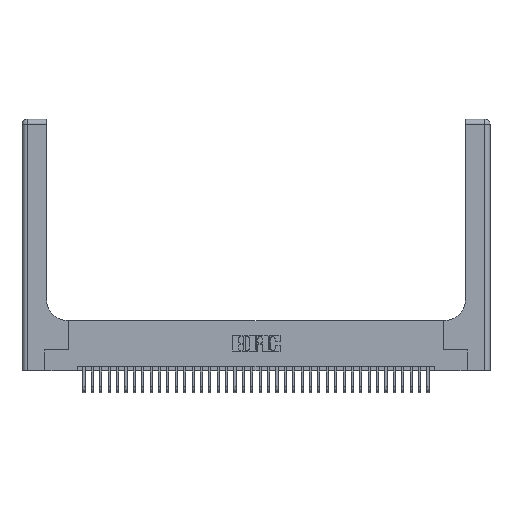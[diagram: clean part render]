
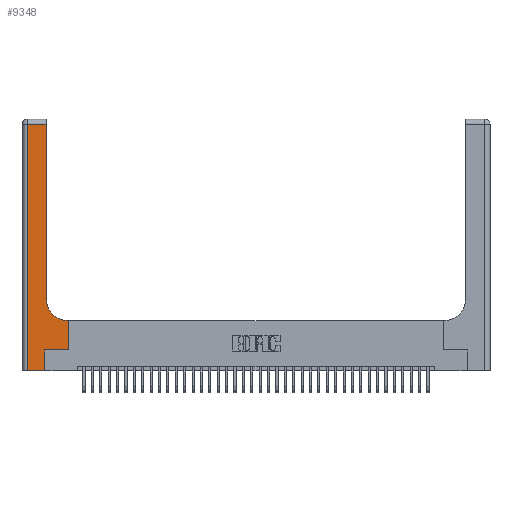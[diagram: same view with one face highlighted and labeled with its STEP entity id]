
A CAD part, top view. The second image highlights one B-rep face of the part: STEP entity #9348.
In plain terms, the highlighted planar face has unit normal (0, 0, 1).
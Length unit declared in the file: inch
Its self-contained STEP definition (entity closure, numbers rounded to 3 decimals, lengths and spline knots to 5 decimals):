
#837 = VECTOR ( 'NONE', #2666, 39.37008 ) ;
#990 = VECTOR ( 'NONE', #32367, 39.37008 ) ;
#1146 = CARTESIAN_POINT ( 'NONE',  ( 0.2915, 0.6, 0.37 ) ) ;
#1640 = CARTESIAN_POINT ( 'NONE',  ( 0., 3., 0.37 ) ) ;
#1773 = DIRECTION ( 'NONE',  ( 0., 0., -1. ) ) ;
#2666 = DIRECTION ( 'NONE',  ( 1., 0., 0. ) ) ;
#3474 = VERTEX_POINT ( 'NONE', #8706 ) ;
#3590 = CARTESIAN_POINT ( 'NONE',  ( 0.269, 0.25, 0.37 ) ) ;
#4107 = ORIENTED_EDGE ( 'NONE', *, *, #10324, .T. ) ;
#4126 = VERTEX_POINT ( 'NONE', #3590 ) ;
#4825 = DIRECTION ( 'NONE',  ( 0., 0., -1. ) ) ;
#5208 = ORIENTED_EDGE ( 'NONE', *, *, #34622, .T. ) ;
#5477 = DIRECTION ( 'NONE',  ( -1., 0., 0. ) ) ;
#5587 = EDGE_CURVE ( 'NONE', #35116, #32030, #19634, .T. ) ;
#6352 = ORIENTED_EDGE ( 'NONE', *, *, #35285, .T. ) ;
#6358 = VECTOR ( 'NONE', #16440, 39.37008 ) ;
#8196 = VECTOR ( 'NONE', #34169, 39.37008 ) ;
#8706 = CARTESIAN_POINT ( 'NONE',  ( 0.06, 2.94, 0.37 ) ) ;
#8717 = EDGE_CURVE ( 'NONE', #3474, #21425, #32733, .T. ) ;
#9348 = ADVANCED_FACE ( 'NONE', ( #12193 ), #35833, .F. ) ;
#9708 = VERTEX_POINT ( 'NONE', #20956 ) ;
#10324 = EDGE_CURVE ( 'NONE', #33354, #25528, #24553, .T. ) ;
#10590 = ORIENTED_EDGE ( 'NONE', *, *, #5587, .T. ) ;
#10992 = CIRCLE ( 'NONE', #30699, 0.25 ) ;
#11014 = VECTOR ( 'NONE', #20987, 39.37008 ) ;
#11579 = LINE ( 'NONE', #24904, #24889 ) ;
#11816 = EDGE_CURVE ( 'NONE', #4126, #33354, #11579, .T. ) ;
#12193 = FACE_OUTER_BOUND ( 'NONE', #32495, .T. ) ;
#12831 = CARTESIAN_POINT ( 'NONE',  ( 0.5585, 0.6, 0.37 ) ) ;
#12863 = CARTESIAN_POINT ( 'NONE',  ( 0.06, 3., 0.37 ) ) ;
#12997 = VERTEX_POINT ( 'NONE', #33874 ) ;
#13680 = LINE ( 'NONE', #36677, #21213 ) ;
#14179 = LINE ( 'NONE', #36724, #837 ) ;
#16154 = EDGE_CURVE ( 'NONE', #12997, #4126, #23298, .T. ) ;
#16440 = DIRECTION ( 'NONE',  ( 0., 1., 0. ) ) ;
#16464 = DIRECTION ( 'NONE',  ( 1., 0., 0. ) ) ;
#16800 = LINE ( 'NONE', #1146, #11014 ) ;
#18146 = CARTESIAN_POINT ( 'NONE',  ( 0.5585, 0.25, 0.37 ) ) ;
#19634 = LINE ( 'NONE', #33490, #6358 ) ;
#19796 = ORIENTED_EDGE ( 'NONE', *, *, #11816, .T. ) ;
#19860 = ORIENTED_EDGE ( 'NONE', *, *, #16154, .T. ) ;
#20956 = CARTESIAN_POINT ( 'NONE',  ( 0.5415, 0.6, 0.37 ) ) ;
#20987 = DIRECTION ( 'NONE',  ( -1., 0., 0. ) ) ;
#21213 = VECTOR ( 'NONE', #5477, 39.37008 ) ;
#21425 = VERTEX_POINT ( 'NONE', #21479 ) ;
#21479 = CARTESIAN_POINT ( 'NONE',  ( 0.06, 0., 0.37 ) ) ;
#21619 = DIRECTION ( 'NONE',  ( -1., 0., 0. ) ) ;
#21792 = CARTESIAN_POINT ( 'NONE',  ( 0.5415, 0.85, 0.37 ) ) ;
#22981 = CARTESIAN_POINT ( 'NONE',  ( 0.2915, 2.94, 0.37 ) ) ;
#23298 = LINE ( 'NONE', #25682, #8196 ) ;
#24168 = DIRECTION ( 'NONE',  ( 0., -1., 0. ) ) ;
#24553 = LINE ( 'NONE', #18146, #990 ) ;
#24662 = DIRECTION ( 'NONE',  ( 1., 0., 0. ) ) ;
#24889 = VECTOR ( 'NONE', #16464, 39.37008 ) ;
#24904 = CARTESIAN_POINT ( 'NONE',  ( 0.269, 0.25, 0.37 ) ) ;
#24922 = EDGE_CURVE ( 'NONE', #9708, #35116, #10992, .T. ) ;
#25528 = VERTEX_POINT ( 'NONE', #12831 ) ;
#25682 = CARTESIAN_POINT ( 'NONE',  ( 0.269, 0., 0.37 ) ) ;
#26904 = ORIENTED_EDGE ( 'NONE', *, *, #31576, .T. ) ;
#27679 = CARTESIAN_POINT ( 'NONE',  ( 0.5585, 0.25, 0.37 ) ) ;
#30699 = AXIS2_PLACEMENT_3D ( 'NONE', #21792, #4825, #24662 ) ;
#31576 = EDGE_CURVE ( 'NONE', #25528, #9708, #16800, .T. ) ;
#32030 = VERTEX_POINT ( 'NONE', #22981 ) ;
#32277 = AXIS2_PLACEMENT_3D ( 'NONE', #1640, #1773, #21619 ) ;
#32367 = DIRECTION ( 'NONE',  ( 0., 1., 0. ) ) ;
#32495 = EDGE_LOOP ( 'NONE', ( #10590, #6352, #33173, #5208, #19860, #19796, #4107, #26904, #35201 ) ) ;
#32733 = LINE ( 'NONE', #12863, #33621 ) ;
#33173 = ORIENTED_EDGE ( 'NONE', *, *, #8717, .T. ) ;
#33354 = VERTEX_POINT ( 'NONE', #27679 ) ;
#33490 = CARTESIAN_POINT ( 'NONE',  ( 0.2915, 3., 0.37 ) ) ;
#33621 = VECTOR ( 'NONE', #24168, 39.37008 ) ;
#33874 = CARTESIAN_POINT ( 'NONE',  ( 0.269, 0., 0.37 ) ) ;
#34169 = DIRECTION ( 'NONE',  ( 0., 1., 0. ) ) ;
#34622 = EDGE_CURVE ( 'NONE', #21425, #12997, #14179, .T. ) ;
#35116 = VERTEX_POINT ( 'NONE', #35796 ) ;
#35201 = ORIENTED_EDGE ( 'NONE', *, *, #24922, .T. ) ;
#35285 = EDGE_CURVE ( 'NONE', #32030, #3474, #13680, .T. ) ;
#35796 = CARTESIAN_POINT ( 'NONE',  ( 0.2915, 0.85, 0.37 ) ) ;
#35833 = PLANE ( 'NONE',  #32277 ) ;
#36677 = CARTESIAN_POINT ( 'NONE',  ( 0., 2.94, 0.37 ) ) ;
#36724 = CARTESIAN_POINT ( 'NONE',  ( 0., 0., 0.37 ) ) ;
